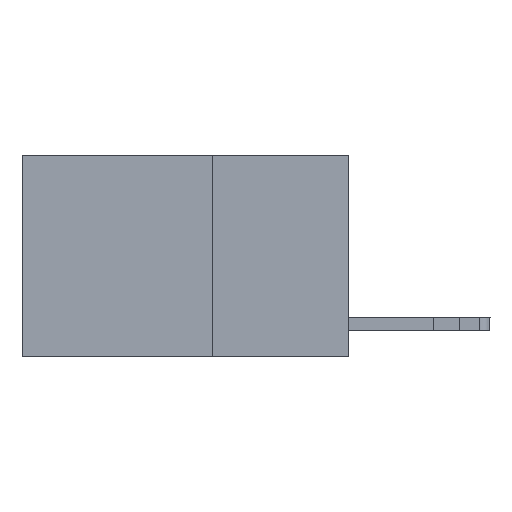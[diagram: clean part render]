
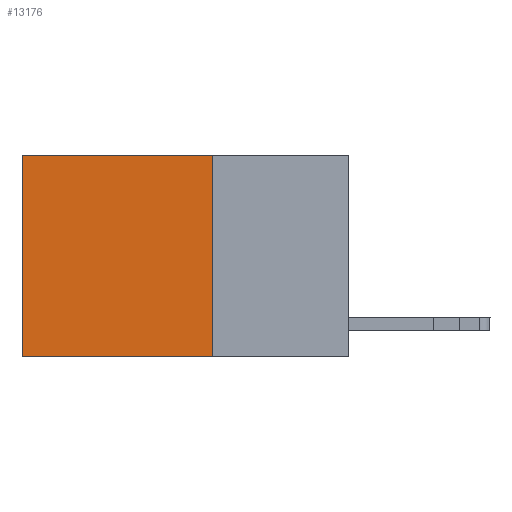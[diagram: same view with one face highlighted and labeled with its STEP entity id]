
A CAD part, left-side view. The second image highlights one B-rep face of the part: STEP entity #13176.
In plain terms, the highlighted planar face has unit normal (-1, 0, 0).
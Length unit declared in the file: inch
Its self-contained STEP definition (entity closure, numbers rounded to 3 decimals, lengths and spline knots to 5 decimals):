
#556 = EDGE_CURVE ( 'NONE', #15406, #6457, #9378, .T. ) ;
#1057 = VERTEX_POINT ( 'NONE', #12974 ) ;
#1449 = ORIENTED_EDGE ( 'NONE', *, *, #556, .F. ) ;
#2247 = EDGE_CURVE ( 'NONE', #6520, #1057, #9303, .T. ) ;
#3006 = PLANE ( 'NONE',  #9189 ) ;
#3044 = LINE ( 'NONE', #8423, #3553 ) ;
#3553 = VECTOR ( 'NONE', #17935, 39.37008 ) ;
#3666 = DIRECTION ( 'NONE',  ( 0., 1., 0. ) ) ;
#4196 = VECTOR ( 'NONE', #3666, 39.37008 ) ;
#4660 = DIRECTION ( 'NONE',  ( 1., 0., 0. ) ) ;
#4932 = ORIENTED_EDGE ( 'NONE', *, *, #6564, .F. ) ;
#5089 = CARTESIAN_POINT ( 'NONE',  ( 0.2625, 0.6, 0. ) ) ;
#5145 = VECTOR ( 'NONE', #13538, 39.37008 ) ;
#5195 = LINE ( 'NONE', #5235, #4196 ) ;
#5235 = CARTESIAN_POINT ( 'NONE',  ( 0.2625, 0.25, -0.37 ) ) ;
#5579 = VECTOR ( 'NONE', #9307, 39.37008 ) ;
#6457 = VERTEX_POINT ( 'NONE', #19177 ) ;
#6520 = VERTEX_POINT ( 'NONE', #5089 ) ;
#6564 = EDGE_CURVE ( 'NONE', #6457, #1057, #5195, .T. ) ;
#6765 = CARTESIAN_POINT ( 'NONE',  ( 0.2625, 0.25, 0. ) ) ;
#8423 = CARTESIAN_POINT ( 'NONE',  ( 0.2625, 0.25, 0. ) ) ;
#8763 = FACE_OUTER_BOUND ( 'NONE', #18655, .T. ) ;
#9189 = AXIS2_PLACEMENT_3D ( 'NONE', #14183, #4660, #15777 ) ;
#9247 = EDGE_CURVE ( 'NONE', #15406, #6520, #3044, .T. ) ;
#9303 = LINE ( 'NONE', #9362, #5579 ) ;
#9307 = DIRECTION ( 'NONE',  ( 0., 0., -1. ) ) ;
#9362 = CARTESIAN_POINT ( 'NONE',  ( 0.2625, 0.6, 0. ) ) ;
#9378 = LINE ( 'NONE', #6765, #5145 ) ;
#10059 = ORIENTED_EDGE ( 'NONE', *, *, #9247, .T. ) ;
#12974 = CARTESIAN_POINT ( 'NONE',  ( 0.2625, 0.6, -0.37 ) ) ;
#13042 = CARTESIAN_POINT ( 'NONE',  ( 0.2625, 0.25, 0. ) ) ;
#13176 = ADVANCED_FACE ( 'NONE', ( #8763 ), #3006, .F. ) ;
#13538 = DIRECTION ( 'NONE',  ( 0., 0., -1. ) ) ;
#14183 = CARTESIAN_POINT ( 'NONE',  ( 0.2625, 0.25, 0. ) ) ;
#15406 = VERTEX_POINT ( 'NONE', #13042 ) ;
#15777 = DIRECTION ( 'NONE',  ( 0., 0., -1. ) ) ;
#17935 = DIRECTION ( 'NONE',  ( 0., 1., 0. ) ) ;
#18192 = ORIENTED_EDGE ( 'NONE', *, *, #2247, .T. ) ;
#18655 = EDGE_LOOP ( 'NONE', ( #18192, #4932, #1449, #10059 ) ) ;
#19177 = CARTESIAN_POINT ( 'NONE',  ( 0.2625, 0.25, -0.37 ) ) ;
